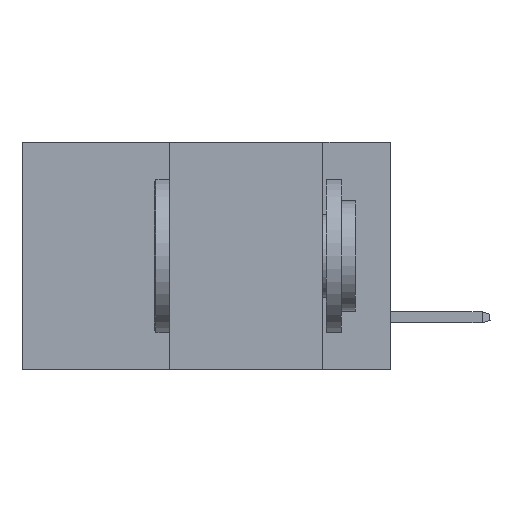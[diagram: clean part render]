
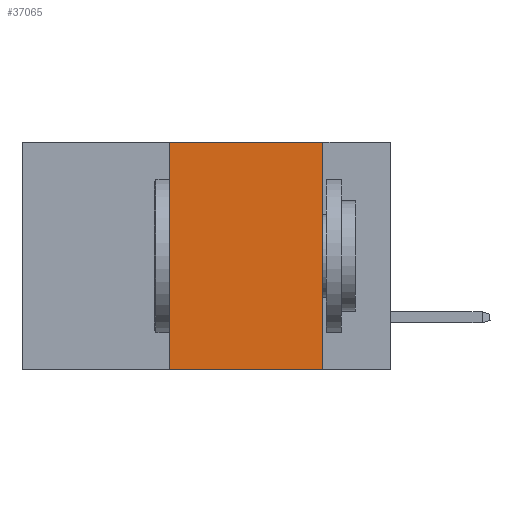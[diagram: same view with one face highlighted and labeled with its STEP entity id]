
A CAD part, left-side view. The second image highlights one B-rep face of the part: STEP entity #37065.
In plain terms, the highlighted planar face has unit normal (-1, 0, 0).
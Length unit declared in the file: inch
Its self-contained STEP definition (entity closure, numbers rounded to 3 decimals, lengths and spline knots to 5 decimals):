
#1937 = VERTEX_POINT ( 'NONE', #16868 ) ;
#2450 = LINE ( 'NONE', #43079, #30123 ) ;
#4406 = ORIENTED_EDGE ( 'NONE', *, *, #6282, .T. ) ;
#6282 = EDGE_CURVE ( 'NONE', #1937, #23067, #11268, .T. ) ;
#8259 = VECTOR ( 'NONE', #14704, 39.37008 ) ;
#8434 = CARTESIAN_POINT ( 'NONE',  ( 0., 0.11, -0.37 ) ) ;
#8954 = CARTESIAN_POINT ( 'NONE',  ( 0., 0.11, 0. ) ) ;
#10542 = LINE ( 'NONE', #25264, #8259 ) ;
#11268 = LINE ( 'NONE', #37878, #38918 ) ;
#12839 = DIRECTION ( 'NONE',  ( 0., 0., -1. ) ) ;
#14291 = DIRECTION ( 'NONE',  ( 0., 0., 1. ) ) ;
#14704 = DIRECTION ( 'NONE',  ( 0., 0., -1. ) ) ;
#15342 = VERTEX_POINT ( 'NONE', #43546 ) ;
#16868 = CARTESIAN_POINT ( 'NONE',  ( 0., 0.36, -0.37 ) ) ;
#17808 = AXIS2_PLACEMENT_3D ( 'NONE', #30836, #45126, #12839 ) ;
#19955 = PLANE ( 'NONE',  #17808 ) ;
#20272 = DIRECTION ( 'NONE',  ( 0., -1., 0. ) ) ;
#21351 = EDGE_LOOP ( 'NONE', ( #30067, #38811, #41134, #4406 ) ) ;
#23067 = VERTEX_POINT ( 'NONE', #8434 ) ;
#23708 = FACE_OUTER_BOUND ( 'NONE', #21351, .T. ) ;
#23754 = VECTOR ( 'NONE', #20272, 39.37008 ) ;
#25264 = CARTESIAN_POINT ( 'NONE',  ( 0., 0.11, 0. ) ) ;
#25992 = DIRECTION ( 'NONE',  ( 0., -1., 0. ) ) ;
#30067 = ORIENTED_EDGE ( 'NONE', *, *, #32167, .F. ) ;
#30123 = VECTOR ( 'NONE', #14291, 39.37008 ) ;
#30836 = CARTESIAN_POINT ( 'NONE',  ( 0., 0.6, 0. ) ) ;
#31085 = LINE ( 'NONE', #31965, #23754 ) ;
#31965 = CARTESIAN_POINT ( 'NONE',  ( 0., 0.6, 0. ) ) ;
#32167 = EDGE_CURVE ( 'NONE', #32427, #23067, #10542, .T. ) ;
#32427 = VERTEX_POINT ( 'NONE', #8954 ) ;
#37065 = ADVANCED_FACE ( 'NONE', ( #23708 ), #19955, .F. ) ;
#37878 = CARTESIAN_POINT ( 'NONE',  ( 0., 0.6, -0.37 ) ) ;
#38811 = ORIENTED_EDGE ( 'NONE', *, *, #42117, .F. ) ;
#38918 = VECTOR ( 'NONE', #25992, 39.37008 ) ;
#41134 = ORIENTED_EDGE ( 'NONE', *, *, #43452, .F. ) ;
#42117 = EDGE_CURVE ( 'NONE', #15342, #32427, #31085, .T. ) ;
#43079 = CARTESIAN_POINT ( 'NONE',  ( 0., 0.36, 0. ) ) ;
#43452 = EDGE_CURVE ( 'NONE', #1937, #15342, #2450, .T. ) ;
#43546 = CARTESIAN_POINT ( 'NONE',  ( 0., 0.36, 0. ) ) ;
#45126 = DIRECTION ( 'NONE',  ( 1., 0., 0. ) ) ;
